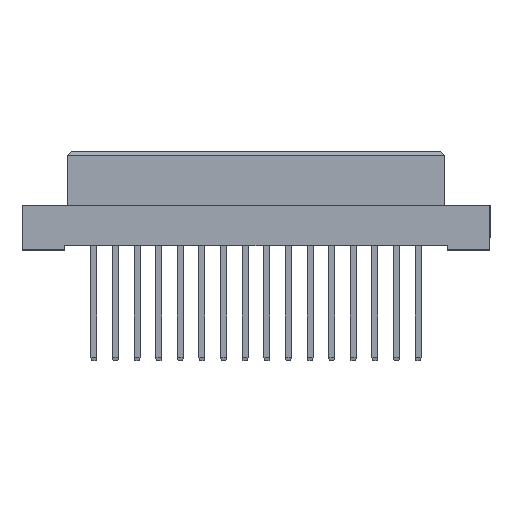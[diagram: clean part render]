
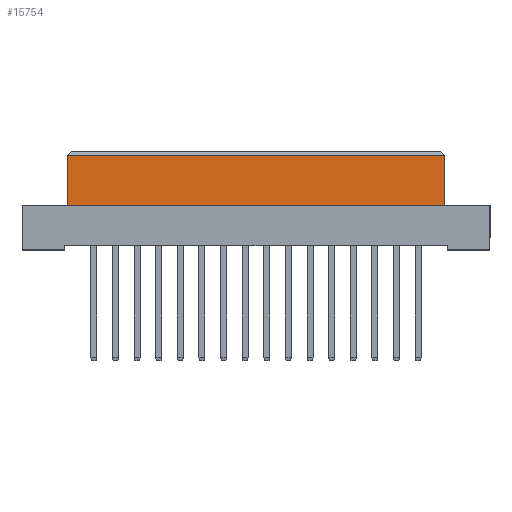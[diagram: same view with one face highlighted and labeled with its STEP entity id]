
A CAD part, top view. The second image highlights one B-rep face of the part: STEP entity #15754.
In plain terms, the highlighted planar face has unit normal (0, 0, 1).
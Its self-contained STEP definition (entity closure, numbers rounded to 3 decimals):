
#157 = CARTESIAN_POINT ( 'NONE',  ( -22.2, -0.5, 4.25 ) ) ;
#729 = DIRECTION ( 'NONE',  ( 0., 1., 0. ) ) ;
#833 = LINE ( 'NONE', #19878, #16556 ) ;
#916 = EDGE_CURVE ( 'NONE', #14731, #20794, #16885, .T. ) ;
#2224 = EDGE_LOOP ( 'NONE', ( #3536, #18287, #19343, #5961 ) ) ;
#2391 = FACE_OUTER_BOUND ( 'NONE', #2224, .T. ) ;
#3536 = ORIENTED_EDGE ( 'NONE', *, *, #5678, .T. ) ;
#4047 = CARTESIAN_POINT ( 'NONE',  ( -22.2, -6.4, 4.25 ) ) ;
#4282 = CARTESIAN_POINT ( 'NONE',  ( 22.2, -6.4, 4.25 ) ) ;
#4365 = DIRECTION ( 'NONE',  ( 1., 0., 0. ) ) ;
#4858 = VECTOR ( 'NONE', #4365, 1000. ) ;
#4888 = VECTOR ( 'NONE', #20041, 1000. ) ;
#5678 = EDGE_CURVE ( 'NONE', #6350, #14731, #833, .T. ) ;
#5690 = CARTESIAN_POINT ( 'NONE',  ( 22.2, -0.5, 4.25 ) ) ;
#5961 = ORIENTED_EDGE ( 'NONE', *, *, #9836, .T. ) ;
#6350 = VERTEX_POINT ( 'NONE', #7330 ) ;
#6678 = EDGE_CURVE ( 'NONE', #17477, #20794, #18677, .T. ) ;
#7314 = LINE ( 'NONE', #7527, #4858 ) ;
#7330 = CARTESIAN_POINT ( 'NONE',  ( 22.2, -6.4, 4.25 ) ) ;
#7420 = AXIS2_PLACEMENT_3D ( 'NONE', #4282, #10694, #12167 ) ;
#7527 = CARTESIAN_POINT ( 'NONE',  ( 22.2, -6.4, 4.25 ) ) ;
#9836 = EDGE_CURVE ( 'NONE', #17477, #6350, #7314, .T. ) ;
#10694 = DIRECTION ( 'NONE',  ( 0., 0., 1. ) ) ;
#12167 = DIRECTION ( 'NONE',  ( 1., 0., 0. ) ) ;
#14046 = DIRECTION ( 'NONE',  ( -1., 0., 0. ) ) ;
#14731 = VERTEX_POINT ( 'NONE', #5690 ) ;
#15295 = CARTESIAN_POINT ( 'NONE',  ( -22.2, -6.4, 4.25 ) ) ;
#15754 = ADVANCED_FACE ( 'NONE', ( #2391 ), #16895, .T. ) ;
#16226 = VECTOR ( 'NONE', #14046, 1000. ) ;
#16556 = VECTOR ( 'NONE', #729, 1000. ) ;
#16885 = LINE ( 'NONE', #17204, #16226 ) ;
#16895 = PLANE ( 'NONE',  #7420 ) ;
#17204 = CARTESIAN_POINT ( 'NONE',  ( -22.2, -0.5, 4.25 ) ) ;
#17477 = VERTEX_POINT ( 'NONE', #4047 ) ;
#18287 = ORIENTED_EDGE ( 'NONE', *, *, #916, .T. ) ;
#18677 = LINE ( 'NONE', #15295, #4888 ) ;
#19343 = ORIENTED_EDGE ( 'NONE', *, *, #6678, .F. ) ;
#19878 = CARTESIAN_POINT ( 'NONE',  ( 22.2, -6.4, 4.25 ) ) ;
#20041 = DIRECTION ( 'NONE',  ( 0., 1., 0. ) ) ;
#20794 = VERTEX_POINT ( 'NONE', #157 ) ;
